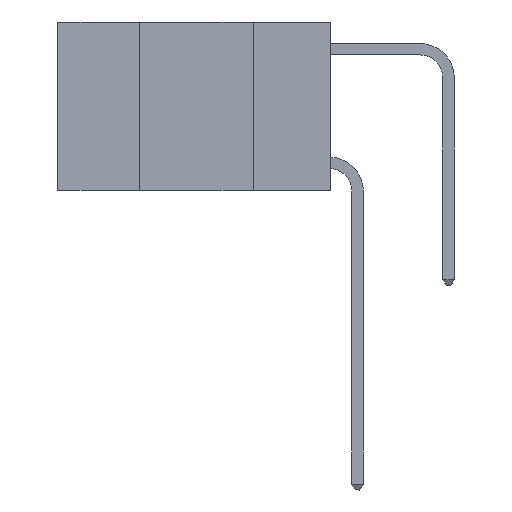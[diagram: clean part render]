
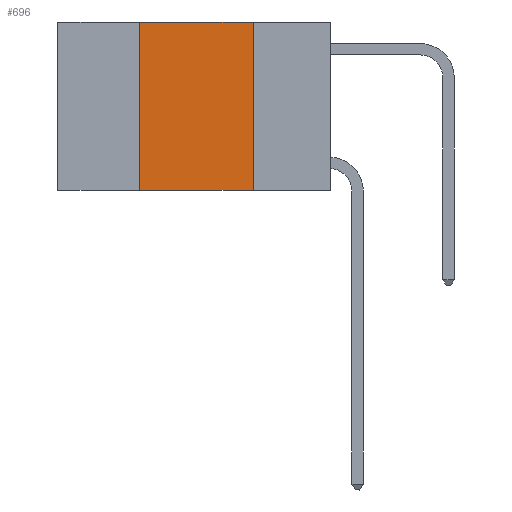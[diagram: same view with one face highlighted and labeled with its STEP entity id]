
A CAD part, left-side view. The second image highlights one B-rep face of the part: STEP entity #696.
In plain terms, the highlighted planar face has unit normal (-1, 0, 0).
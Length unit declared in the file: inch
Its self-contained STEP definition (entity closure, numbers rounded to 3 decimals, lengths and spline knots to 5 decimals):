
#235 = CARTESIAN_POINT ( 'NONE',  ( 0., 0.42, 0. ) ) ;
#696 = ADVANCED_FACE ( 'NONE', ( #18846 ), #1211, .F. ) ;
#1211 = PLANE ( 'NONE',  #10998 ) ;
#1858 = CARTESIAN_POINT ( 'NONE',  ( 0., 0.17, 0. ) ) ;
#1957 = EDGE_CURVE ( 'NONE', #13040, #18875, #12218, .T. ) ;
#2029 = ORIENTED_EDGE ( 'NONE', *, *, #5413, .F. ) ;
#2640 = EDGE_LOOP ( 'NONE', ( #2029, #10175, #18191, #18667 ) ) ;
#2732 = DIRECTION ( 'NONE',  ( 1., 0., 0. ) ) ;
#4861 = VERTEX_POINT ( 'NONE', #10176 ) ;
#5124 = CARTESIAN_POINT ( 'NONE',  ( 0., 0.6, -0.37 ) ) ;
#5413 = EDGE_CURVE ( 'NONE', #17954, #4861, #11283, .T. ) ;
#5495 = CARTESIAN_POINT ( 'NONE',  ( 0., 0.42, 0. ) ) ;
#5655 = DIRECTION ( 'NONE',  ( 0., 0., -1. ) ) ;
#7086 = CARTESIAN_POINT ( 'NONE',  ( 0., 0.6, 0. ) ) ;
#8140 = VECTOR ( 'NONE', #14654, 39.37008 ) ;
#8199 = EDGE_CURVE ( 'NONE', #18875, #17954, #19428, .T. ) ;
#9876 = VECTOR ( 'NONE', #12832, 39.37008 ) ;
#10175 = ORIENTED_EDGE ( 'NONE', *, *, #8199, .F. ) ;
#10176 = CARTESIAN_POINT ( 'NONE',  ( 0., 0.17, -0.37 ) ) ;
#10802 = VECTOR ( 'NONE', #5655, 39.37008 ) ;
#10998 = AXIS2_PLACEMENT_3D ( 'NONE', #14892, #2732, #13444 ) ;
#11283 = LINE ( 'NONE', #14815, #10802 ) ;
#12218 = LINE ( 'NONE', #5495, #8140 ) ;
#12459 = CARTESIAN_POINT ( 'NONE',  ( 0., 0.42, -0.37 ) ) ;
#12832 = DIRECTION ( 'NONE',  ( 0., -1., 0. ) ) ;
#13040 = VERTEX_POINT ( 'NONE', #12459 ) ;
#13444 = DIRECTION ( 'NONE',  ( 0., 0., -1. ) ) ;
#13873 = EDGE_CURVE ( 'NONE', #13040, #4861, #13928, .T. ) ;
#13928 = LINE ( 'NONE', #5124, #9876 ) ;
#14654 = DIRECTION ( 'NONE',  ( 0., 0., 1. ) ) ;
#14706 = DIRECTION ( 'NONE',  ( 0., -1., 0. ) ) ;
#14815 = CARTESIAN_POINT ( 'NONE',  ( 0., 0.17, 0. ) ) ;
#14892 = CARTESIAN_POINT ( 'NONE',  ( 0., 0.6, 0. ) ) ;
#16394 = VECTOR ( 'NONE', #14706, 39.37008 ) ;
#17954 = VERTEX_POINT ( 'NONE', #1858 ) ;
#18191 = ORIENTED_EDGE ( 'NONE', *, *, #1957, .F. ) ;
#18667 = ORIENTED_EDGE ( 'NONE', *, *, #13873, .T. ) ;
#18846 = FACE_OUTER_BOUND ( 'NONE', #2640, .T. ) ;
#18875 = VERTEX_POINT ( 'NONE', #235 ) ;
#19428 = LINE ( 'NONE', #7086, #16394 ) ;
